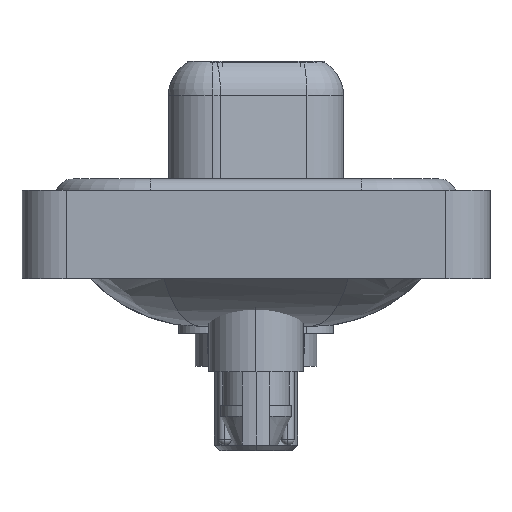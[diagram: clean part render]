
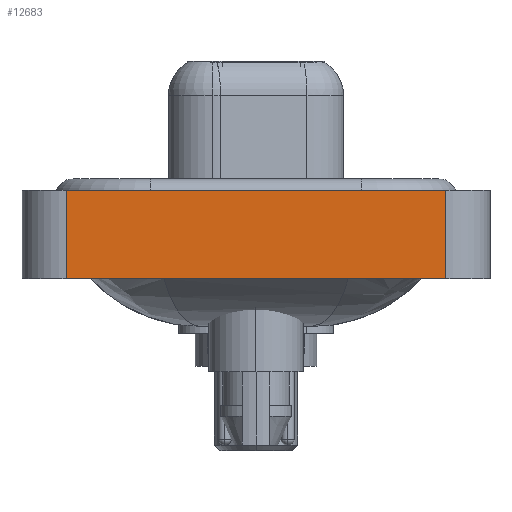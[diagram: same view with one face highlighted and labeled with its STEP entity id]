
A CAD part, left-side view. The second image highlights one B-rep face of the part: STEP entity #12683.
In plain terms, the highlighted planar face has unit normal (-1, 0, 0).
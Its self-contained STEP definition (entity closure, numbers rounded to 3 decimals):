
#88 = DIRECTION ( 'NONE',  ( 0., 0., 1. ) ) ;
#109 = DIRECTION ( 'NONE',  ( -1., 0., 0. ) ) ;
#360 = VECTOR ( 'NONE', #10521, 1000. ) ;
#982 = CARTESIAN_POINT ( 'NONE',  ( -7.35, 8.55, 0.4 ) ) ;
#1266 = VERTEX_POINT ( 'NONE', #16629 ) ;
#2413 = CARTESIAN_POINT ( 'NONE',  ( -7.35, -8.55, 0.4 ) ) ;
#4014 = EDGE_CURVE ( 'NONE', #1266, #17991, #12111, .T. ) ;
#4369 = LINE ( 'NONE', #16524, #360 ) ;
#5138 = ORIENTED_EDGE ( 'NONE', *, *, #13857, .F. ) ;
#5404 = VERTEX_POINT ( 'NONE', #25457 ) ;
#5586 = LINE ( 'NONE', #21033, #14031 ) ;
#6128 = AXIS2_PLACEMENT_3D ( 'NONE', #8311, #109, #18973 ) ;
#7027 = ORIENTED_EDGE ( 'NONE', *, *, #11940, .F. ) ;
#8311 = CARTESIAN_POINT ( 'NONE',  ( -7.35, -8.55, -3.6 ) ) ;
#10521 = DIRECTION ( 'NONE',  ( 0., -1., 0. ) ) ;
#11940 = EDGE_CURVE ( 'NONE', #5404, #24069, #14499, .T. ) ;
#12111 = LINE ( 'NONE', #21009, #23800 ) ;
#12683 = ADVANCED_FACE ( 'NONE', ( #14440 ), #18840, .T. ) ;
#13538 = EDGE_LOOP ( 'NONE', ( #17545, #5138, #7027, #21122 ) ) ;
#13857 = EDGE_CURVE ( 'NONE', #24069, #17991, #5586, .T. ) ;
#14031 = VECTOR ( 'NONE', #21162, 1000. ) ;
#14440 = FACE_OUTER_BOUND ( 'NONE', #13538, .T. ) ;
#14499 = LINE ( 'NONE', #26955, #15238 ) ;
#15238 = VECTOR ( 'NONE', #16568, 1000. ) ;
#16524 = CARTESIAN_POINT ( 'NONE',  ( -7.35, -8.55, -3.6 ) ) ;
#16568 = DIRECTION ( 'NONE',  ( 0., 0., 1. ) ) ;
#16629 = CARTESIAN_POINT ( 'NONE',  ( -7.35, -8.55, -3.6 ) ) ;
#17545 = ORIENTED_EDGE ( 'NONE', *, *, #4014, .T. ) ;
#17991 = VERTEX_POINT ( 'NONE', #2413 ) ;
#18840 = PLANE ( 'NONE',  #6128 ) ;
#18973 = DIRECTION ( 'NONE',  ( 0., 0., 1. ) ) ;
#21009 = CARTESIAN_POINT ( 'NONE',  ( -7.35, -8.55, -3.6 ) ) ;
#21033 = CARTESIAN_POINT ( 'NONE',  ( -7.35, -8.55, 0.4 ) ) ;
#21122 = ORIENTED_EDGE ( 'NONE', *, *, #23009, .T. ) ;
#21162 = DIRECTION ( 'NONE',  ( 0., -1., 0. ) ) ;
#23009 = EDGE_CURVE ( 'NONE', #5404, #1266, #4369, .T. ) ;
#23800 = VECTOR ( 'NONE', #88, 1000. ) ;
#24069 = VERTEX_POINT ( 'NONE', #982 ) ;
#25457 = CARTESIAN_POINT ( 'NONE',  ( -7.35, 8.55, -3.6 ) ) ;
#26955 = CARTESIAN_POINT ( 'NONE',  ( -7.35, 8.55, -3.6 ) ) ;
